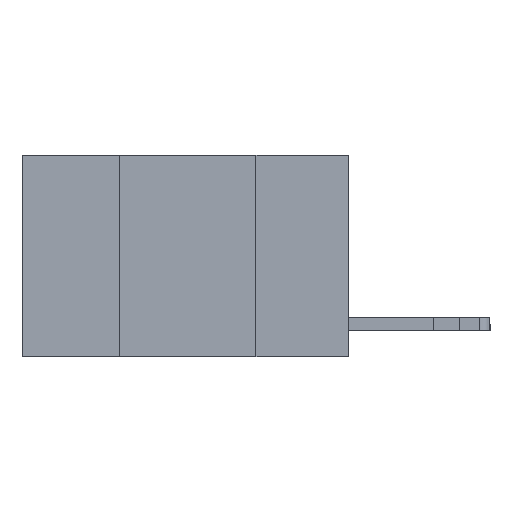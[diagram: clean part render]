
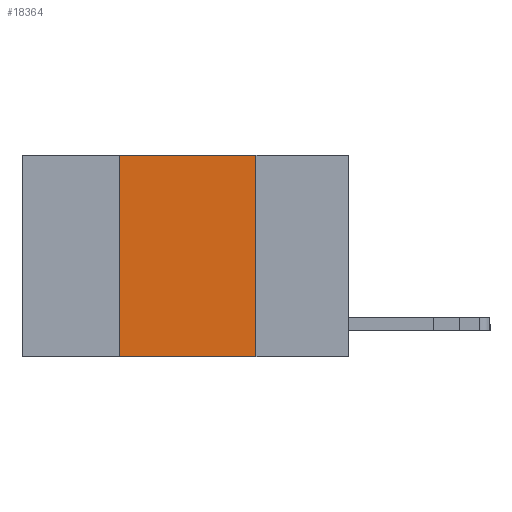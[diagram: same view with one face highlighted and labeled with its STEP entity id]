
A CAD part, left-side view. The second image highlights one B-rep face of the part: STEP entity #18364.
In plain terms, the highlighted planar face has unit normal (-1, 0, 0).
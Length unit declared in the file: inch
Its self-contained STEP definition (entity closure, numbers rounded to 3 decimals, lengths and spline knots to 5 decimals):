
#545 = VERTEX_POINT ( 'NONE', #17633 ) ;
#1122 = VERTEX_POINT ( 'NONE', #9740 ) ;
#1914 = DIRECTION ( 'NONE',  ( 0., -1., 0. ) ) ;
#3103 = CARTESIAN_POINT ( 'NONE',  ( 0., 0.17, -0.37 ) ) ;
#3404 = CARTESIAN_POINT ( 'NONE',  ( 0., 0.17, 0. ) ) ;
#4154 = EDGE_CURVE ( 'NONE', #545, #22796, #17822, .T. ) ;
#4844 = ORIENTED_EDGE ( 'NONE', *, *, #23348, .F. ) ;
#5284 = DIRECTION ( 'NONE',  ( 0., 0., -1. ) ) ;
#5919 = VECTOR ( 'NONE', #9138, 39.37008 ) ;
#6386 = ORIENTED_EDGE ( 'NONE', *, *, #4154, .F. ) ;
#8718 = EDGE_CURVE ( 'NONE', #545, #13659, #14747, .T. ) ;
#8986 = FACE_OUTER_BOUND ( 'NONE', #16891, .T. ) ;
#9138 = DIRECTION ( 'NONE',  ( 0., 0., -1. ) ) ;
#9676 = VECTOR ( 'NONE', #12655, 39.37008 ) ;
#9740 = CARTESIAN_POINT ( 'NONE',  ( 0., 0.17, 0. ) ) ;
#9744 = CARTESIAN_POINT ( 'NONE',  ( 0., 0.6, -0.37 ) ) ;
#9780 = ORIENTED_EDGE ( 'NONE', *, *, #22134, .F. ) ;
#12166 = CARTESIAN_POINT ( 'NONE',  ( 0., 0.42, 0. ) ) ;
#12655 = DIRECTION ( 'NONE',  ( 0., 0., 1. ) ) ;
#12953 = PLANE ( 'NONE',  #16331 ) ;
#13659 = VERTEX_POINT ( 'NONE', #3103 ) ;
#14434 = CARTESIAN_POINT ( 'NONE',  ( 0., 0.6, 0. ) ) ;
#14747 = LINE ( 'NONE', #9744, #23339 ) ;
#14795 = LINE ( 'NONE', #14434, #22328 ) ;
#16331 = AXIS2_PLACEMENT_3D ( 'NONE', #21723, #19913, #5284 ) ;
#16891 = EDGE_LOOP ( 'NONE', ( #4844, #9780, #6386, #23285 ) ) ;
#17633 = CARTESIAN_POINT ( 'NONE',  ( 0., 0.42, -0.37 ) ) ;
#17822 = LINE ( 'NONE', #19855, #9676 ) ;
#18364 = ADVANCED_FACE ( 'NONE', ( #8986 ), #12953, .F. ) ;
#19855 = CARTESIAN_POINT ( 'NONE',  ( 0., 0.42, 0. ) ) ;
#19913 = DIRECTION ( 'NONE',  ( 1., 0., 0. ) ) ;
#21723 = CARTESIAN_POINT ( 'NONE',  ( 0., 0.6, 0. ) ) ;
#21753 = DIRECTION ( 'NONE',  ( 0., -1., 0. ) ) ;
#21757 = LINE ( 'NONE', #3404, #5919 ) ;
#22134 = EDGE_CURVE ( 'NONE', #22796, #1122, #14795, .T. ) ;
#22328 = VECTOR ( 'NONE', #21753, 39.37008 ) ;
#22796 = VERTEX_POINT ( 'NONE', #12166 ) ;
#23285 = ORIENTED_EDGE ( 'NONE', *, *, #8718, .T. ) ;
#23339 = VECTOR ( 'NONE', #1914, 39.37008 ) ;
#23348 = EDGE_CURVE ( 'NONE', #1122, #13659, #21757, .T. ) ;
